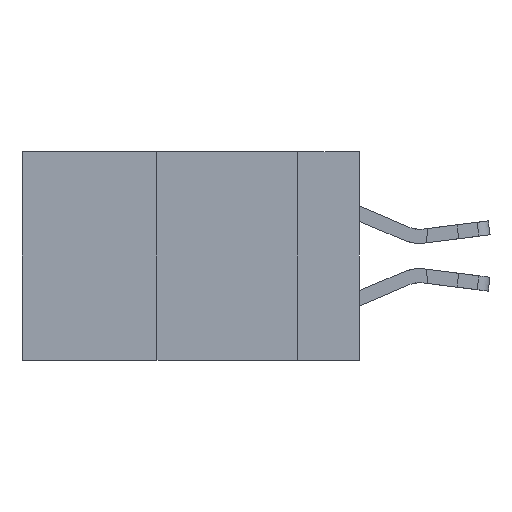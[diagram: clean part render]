
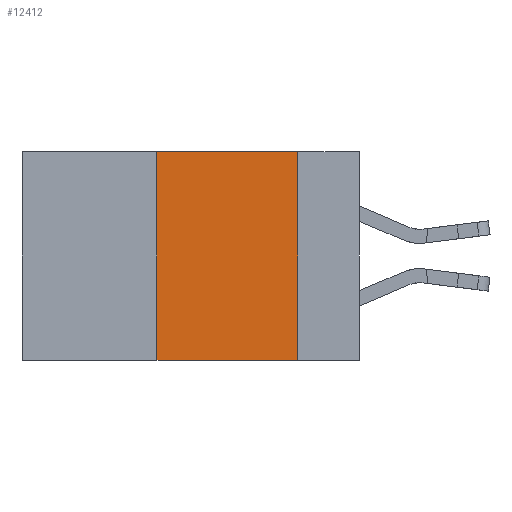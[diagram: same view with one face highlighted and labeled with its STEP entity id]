
A CAD part, left-side view. The second image highlights one B-rep face of the part: STEP entity #12412.
In plain terms, the highlighted planar face has unit normal (-1, 0, 0).
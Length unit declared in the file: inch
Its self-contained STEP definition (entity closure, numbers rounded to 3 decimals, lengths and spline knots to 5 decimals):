
#233 = CARTESIAN_POINT ( 'NONE',  ( 0., 0.36, 0. ) ) ;
#283 = LINE ( 'NONE', #820, #14742 ) ;
#820 = CARTESIAN_POINT ( 'NONE',  ( 0., 0.11, 0. ) ) ;
#2079 = CARTESIAN_POINT ( 'NONE',  ( 0., 0.6, 0. ) ) ;
#2467 = DIRECTION ( 'NONE',  ( 0., 0., -1. ) ) ;
#3559 = VECTOR ( 'NONE', #18362, 39.37008 ) ;
#3825 = LINE ( 'NONE', #15801, #3559 ) ;
#3859 = CARTESIAN_POINT ( 'NONE',  ( 0., 0.6, 0. ) ) ;
#3963 = CARTESIAN_POINT ( 'NONE',  ( 0., 0.11, -0.37 ) ) ;
#4853 = EDGE_LOOP ( 'NONE', ( #19255, #9102, #6474, #14862 ) ) ;
#5202 = EDGE_CURVE ( 'NONE', #5424, #13721, #3825, .T. ) ;
#5424 = VERTEX_POINT ( 'NONE', #15224 ) ;
#5621 = PLANE ( 'NONE',  #7822 ) ;
#6474 = ORIENTED_EDGE ( 'NONE', *, *, #5202, .F. ) ;
#7003 = EDGE_CURVE ( 'NONE', #14601, #17155, #283, .T. ) ;
#7822 = AXIS2_PLACEMENT_3D ( 'NONE', #3859, #20153, #15207 ) ;
#8672 = CARTESIAN_POINT ( 'NONE',  ( 0., 0.11, 0. ) ) ;
#9097 = VECTOR ( 'NONE', #9771, 39.37008 ) ;
#9102 = ORIENTED_EDGE ( 'NONE', *, *, #17097, .F. ) ;
#9771 = DIRECTION ( 'NONE',  ( 0., -1., 0. ) ) ;
#10865 = LINE ( 'NONE', #14113, #9097 ) ;
#11371 = VECTOR ( 'NONE', #13334, 39.37008 ) ;
#12412 = ADVANCED_FACE ( 'NONE', ( #15095 ), #5621, .F. ) ;
#13334 = DIRECTION ( 'NONE',  ( 0., -1., 0. ) ) ;
#13721 = VERTEX_POINT ( 'NONE', #233 ) ;
#14113 = CARTESIAN_POINT ( 'NONE',  ( 0., 0.6, -0.37 ) ) ;
#14601 = VERTEX_POINT ( 'NONE', #8672 ) ;
#14742 = VECTOR ( 'NONE', #2467, 39.37008 ) ;
#14862 = ORIENTED_EDGE ( 'NONE', *, *, #17402, .T. ) ;
#15095 = FACE_OUTER_BOUND ( 'NONE', #4853, .T. ) ;
#15207 = DIRECTION ( 'NONE',  ( 0., 0., -1. ) ) ;
#15224 = CARTESIAN_POINT ( 'NONE',  ( 0., 0.36, -0.37 ) ) ;
#15801 = CARTESIAN_POINT ( 'NONE',  ( 0., 0.36, 0. ) ) ;
#16170 = LINE ( 'NONE', #2079, #11371 ) ;
#17097 = EDGE_CURVE ( 'NONE', #13721, #14601, #16170, .T. ) ;
#17155 = VERTEX_POINT ( 'NONE', #3963 ) ;
#17402 = EDGE_CURVE ( 'NONE', #5424, #17155, #10865, .T. ) ;
#18362 = DIRECTION ( 'NONE',  ( 0., 0., 1. ) ) ;
#19255 = ORIENTED_EDGE ( 'NONE', *, *, #7003, .F. ) ;
#20153 = DIRECTION ( 'NONE',  ( 1., 0., 0. ) ) ;
